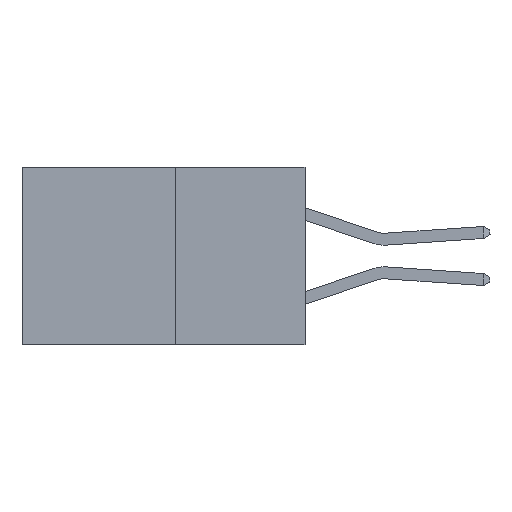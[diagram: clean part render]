
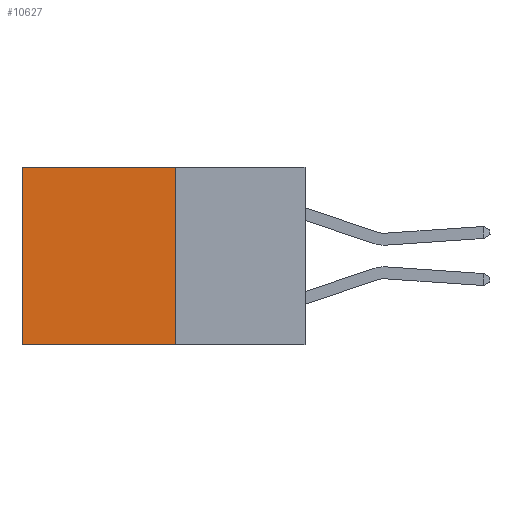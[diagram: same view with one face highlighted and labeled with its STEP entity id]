
A CAD part, left-side view. The second image highlights one B-rep face of the part: STEP entity #10627.
In plain terms, the highlighted planar face has unit normal (-1, 0, 0).
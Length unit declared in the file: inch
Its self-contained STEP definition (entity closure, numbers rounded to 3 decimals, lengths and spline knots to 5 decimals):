
#166 = DIRECTION ( 'NONE',  ( 0., 1., 0. ) ) ;
#377 = LINE ( 'NONE', #13143, #12606 ) ;
#1671 = AXIS2_PLACEMENT_3D ( 'NONE', #14056, #7157, #15225 ) ;
#2358 = FACE_OUTER_BOUND ( 'NONE', #4292, .T. ) ;
#2474 = EDGE_CURVE ( 'NONE', #2664, #4267, #8757, .T. ) ;
#2664 = VERTEX_POINT ( 'NONE', #15166 ) ;
#3122 = CARTESIAN_POINT ( 'NONE',  ( 0.277, 0.59, -0.37 ) ) ;
#3226 = ORIENTED_EDGE ( 'NONE', *, *, #6579, .F. ) ;
#4267 = VERTEX_POINT ( 'NONE', #6369 ) ;
#4292 = EDGE_LOOP ( 'NONE', ( #11362, #3226, #9754, #10106 ) ) ;
#5470 = VECTOR ( 'NONE', #5973, 39.37008 ) ;
#5668 = VECTOR ( 'NONE', #9746, 39.37008 ) ;
#5847 = LINE ( 'NONE', #5924, #5470 ) ;
#5924 = CARTESIAN_POINT ( 'NONE',  ( 0.277, 0.27, -0.37 ) ) ;
#5973 = DIRECTION ( 'NONE',  ( 0., 0., -1. ) ) ;
#5983 = PLANE ( 'NONE',  #1671 ) ;
#6021 = VERTEX_POINT ( 'NONE', #13427 ) ;
#6369 = CARTESIAN_POINT ( 'NONE',  ( 0.277, 0.59, -0.37 ) ) ;
#6579 = EDGE_CURVE ( 'NONE', #11998, #4267, #11986, .T. ) ;
#7157 = DIRECTION ( 'NONE',  ( 1., 0., 0. ) ) ;
#8240 = EDGE_CURVE ( 'NONE', #6021, #11998, #5847, .T. ) ;
#8745 = CARTESIAN_POINT ( 'NONE',  ( 0.277, 0.27, -0.37 ) ) ;
#8757 = LINE ( 'NONE', #3122, #5668 ) ;
#8842 = DIRECTION ( 'NONE',  ( 0., 1., 0. ) ) ;
#9129 = CARTESIAN_POINT ( 'NONE',  ( 0.277, 0.27, -0.37 ) ) ;
#9746 = DIRECTION ( 'NONE',  ( 0., 0., -1. ) ) ;
#9754 = ORIENTED_EDGE ( 'NONE', *, *, #8240, .F. ) ;
#10106 = ORIENTED_EDGE ( 'NONE', *, *, #10772, .T. ) ;
#10627 = ADVANCED_FACE ( 'NONE', ( #2358 ), #5983, .F. ) ;
#10772 = EDGE_CURVE ( 'NONE', #6021, #2664, #377, .T. ) ;
#11362 = ORIENTED_EDGE ( 'NONE', *, *, #2474, .T. ) ;
#11986 = LINE ( 'NONE', #9129, #14779 ) ;
#11998 = VERTEX_POINT ( 'NONE', #8745 ) ;
#12606 = VECTOR ( 'NONE', #166, 39.37008 ) ;
#13143 = CARTESIAN_POINT ( 'NONE',  ( 0.277, 0.27, 0. ) ) ;
#13427 = CARTESIAN_POINT ( 'NONE',  ( 0.277, 0.27, 0. ) ) ;
#14056 = CARTESIAN_POINT ( 'NONE',  ( 0.277, 0.27, -0.37 ) ) ;
#14779 = VECTOR ( 'NONE', #8842, 39.37008 ) ;
#15166 = CARTESIAN_POINT ( 'NONE',  ( 0.277, 0.59, 0. ) ) ;
#15225 = DIRECTION ( 'NONE',  ( 0., 0., -1. ) ) ;
